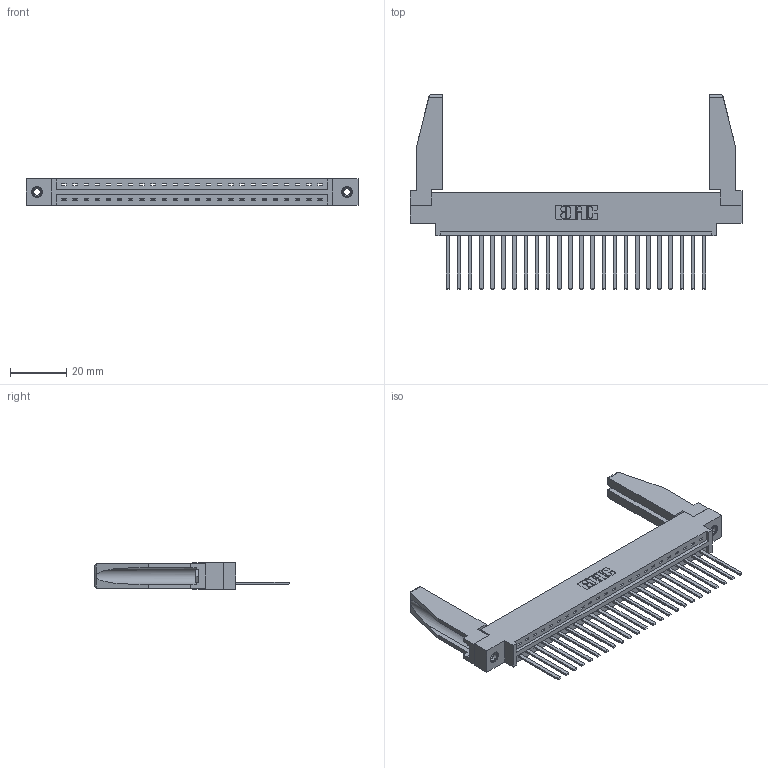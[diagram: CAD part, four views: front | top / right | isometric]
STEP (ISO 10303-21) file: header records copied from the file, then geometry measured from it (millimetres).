
FILE_DESCRIPTION (( 'STEP AP203' ), '1' );
FILE_NAME ('337-024-544-678.STEP', '2019-09-30T16:10:58', ( '' ), ( '' ), 'SwSTEP 2.0', 'SolidWorks 2016', '' );
FILE_SCHEMA (( 'CONFIG_CONTROL_DESIGN' ));
Length unit declared in the file: inch
Products named in the file (5): 337 Part_0.170 Offset - 0.156 Dia-TI; 337-024-544-678; 307-220-078; 345-250-001_345-250-001-102; 345-292-001_345-293-144
Assembly tree (29 placements, depth 2):
  337-024-544-678
    337 Part_0.170 Offset - 0.156 Dia-TI
    345-292-001_345-293-144  x24
    345-250-001_345-250-001-102  x2
    307-220-078  x2
Bounding box: 118.11 x 69.09 x 9.4 mm (x, y, z)
Volume: 16204.1 mm3; surface area: 17365.8 mm2
Topology: 29 solids, 29 shells, 1592 faces, 4733 edges, 3114 vertices
Faces by surface type: plane 1166, cylinder 410, cone 12, torus 4
Entity records: 22556 total; most frequent: CARTESIAN_POINT 3920, ORIENTED_EDGE 3836, DIRECTION 3342, EDGE_CURVE 1918, LINE 1756, VECTOR 1756, VERTEX_POINT 1272, AXIS2_PLACEMENT_3D 793
